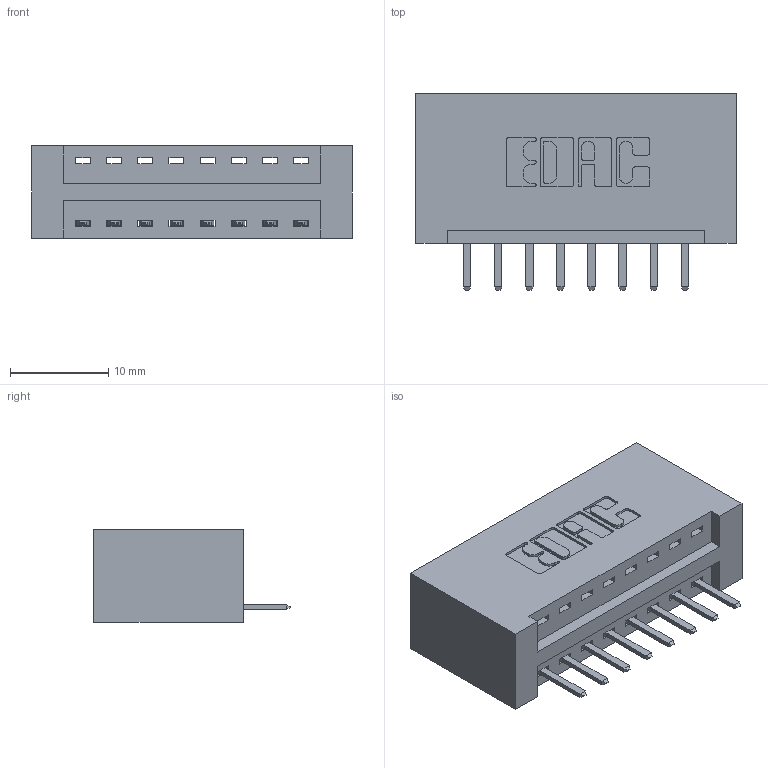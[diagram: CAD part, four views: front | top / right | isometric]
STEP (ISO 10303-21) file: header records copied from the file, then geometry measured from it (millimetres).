
FILE_DESCRIPTION (( 'STEP AP203' ), '1' );
FILE_NAME ('396-008-520-101.STEP', '2019-10-25T18:32:46', ( '' ), ( '' ), 'SwSTEP 2.0', 'SolidWorks 2016', '' );
FILE_SCHEMA (( 'CONFIG_CONTROL_DESIGN' ));
Length unit declared in the file: inch
Products named in the file (3): 396-008-520-101; 345-292-001_345-293-120; 346 Part_No Mounting Lugs
Assembly tree (9 placements, depth 2):
  396-008-520-101
    346 Part_No Mounting Lugs
    345-292-001_345-293-120  x8
Bounding box: 32.64 x 20.02 x 9.4 mm (x, y, z)
Volume: 3416.4 mm3; surface area: 3901.5 mm2
Topology: 9 solids, 9 shells, 610 faces, 1777 edges, 1162 vertices
Faces by surface type: plane 408, cylinder 202
Entity records: 9379 total; most frequent: CARTESIAN_POINT 1636, ORIENTED_EDGE 1566, DIRECTION 1467, EDGE_CURVE 783, VECTOR 623, LINE 623, VERTEX_POINT 518, AXIS2_PLACEMENT_3D 422
